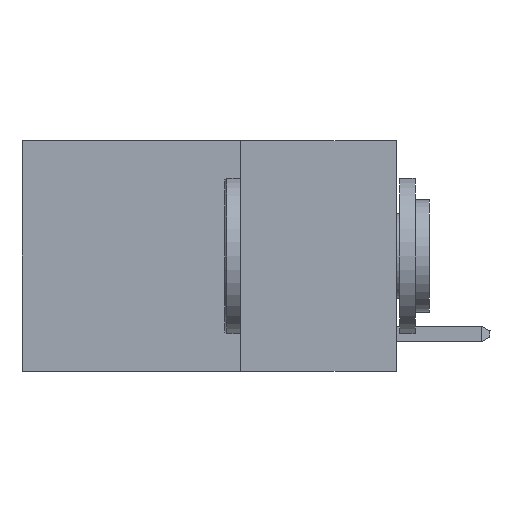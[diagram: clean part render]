
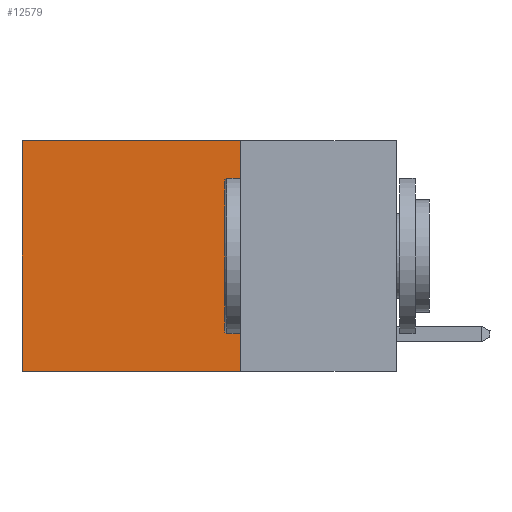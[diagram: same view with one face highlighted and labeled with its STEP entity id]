
A CAD part, left-side view. The second image highlights one B-rep face of the part: STEP entity #12579.
In plain terms, the highlighted planar face has unit normal (-1, 0, 0).
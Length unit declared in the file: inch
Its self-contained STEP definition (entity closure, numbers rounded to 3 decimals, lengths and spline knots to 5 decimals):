
#17 = ORIENTED_EDGE ( 'NONE', *, *, #12261, .F. ) ;
#69 = VERTEX_POINT ( 'NONE', #8329 ) ;
#309 = DIRECTION ( 'NONE',  ( 0., 1., 0. ) ) ;
#559 = DIRECTION ( 'NONE',  ( 0., 1., 0. ) ) ;
#824 = LINE ( 'NONE', #8284, #10235 ) ;
#1229 = VECTOR ( 'NONE', #559, 39.37008 ) ;
#1463 = VERTEX_POINT ( 'NONE', #1734 ) ;
#1734 = CARTESIAN_POINT ( 'NONE',  ( 0.2625, 0.25, -0.37 ) ) ;
#2022 = LINE ( 'NONE', #13952, #13651 ) ;
#2946 = EDGE_CURVE ( 'NONE', #6722, #69, #2022, .T. ) ;
#3266 = DIRECTION ( 'NONE',  ( 0., 0., -1. ) ) ;
#3335 = FACE_OUTER_BOUND ( 'NONE', #5628, .T. ) ;
#3729 = AXIS2_PLACEMENT_3D ( 'NONE', #11222, #13467, #6770 ) ;
#4528 = VERTEX_POINT ( 'NONE', #11102 ) ;
#4775 = ORIENTED_EDGE ( 'NONE', *, *, #5947, .F. ) ;
#4796 = ORIENTED_EDGE ( 'NONE', *, *, #7367, .T. ) ;
#5622 = PLANE ( 'NONE',  #3729 ) ;
#5628 = EDGE_LOOP ( 'NONE', ( #7442, #17, #4775, #4796 ) ) ;
#5947 = EDGE_CURVE ( 'NONE', #4528, #1463, #8148, .T. ) ;
#6650 = CARTESIAN_POINT ( 'NONE',  ( 0.2625, 0.25, 0. ) ) ;
#6722 = VERTEX_POINT ( 'NONE', #10455 ) ;
#6770 = DIRECTION ( 'NONE',  ( 0., 0., -1. ) ) ;
#7084 = VECTOR ( 'NONE', #3266, 39.37008 ) ;
#7367 = EDGE_CURVE ( 'NONE', #4528, #6722, #824, .T. ) ;
#7384 = CARTESIAN_POINT ( 'NONE',  ( 0.2625, 0.25, -0.37 ) ) ;
#7442 = ORIENTED_EDGE ( 'NONE', *, *, #2946, .T. ) ;
#8148 = LINE ( 'NONE', #6650, #7084 ) ;
#8284 = CARTESIAN_POINT ( 'NONE',  ( 0.2625, 0.25, 0. ) ) ;
#8329 = CARTESIAN_POINT ( 'NONE',  ( 0.2625, 0.6, -0.37 ) ) ;
#9597 = LINE ( 'NONE', #7384, #1229 ) ;
#10235 = VECTOR ( 'NONE', #309, 39.37008 ) ;
#10455 = CARTESIAN_POINT ( 'NONE',  ( 0.2625, 0.6, 0. ) ) ;
#10638 = DIRECTION ( 'NONE',  ( 0., 0., -1. ) ) ;
#11102 = CARTESIAN_POINT ( 'NONE',  ( 0.2625, 0.25, 0. ) ) ;
#11222 = CARTESIAN_POINT ( 'NONE',  ( 0.2625, 0.25, 0. ) ) ;
#12261 = EDGE_CURVE ( 'NONE', #1463, #69, #9597, .T. ) ;
#12579 = ADVANCED_FACE ( 'NONE', ( #3335 ), #5622, .F. ) ;
#13467 = DIRECTION ( 'NONE',  ( 1., 0., 0. ) ) ;
#13651 = VECTOR ( 'NONE', #10638, 39.37008 ) ;
#13952 = CARTESIAN_POINT ( 'NONE',  ( 0.2625, 0.6, 0. ) ) ;
